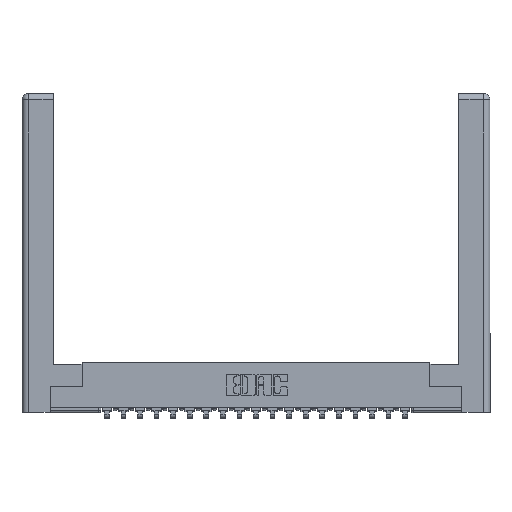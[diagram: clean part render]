
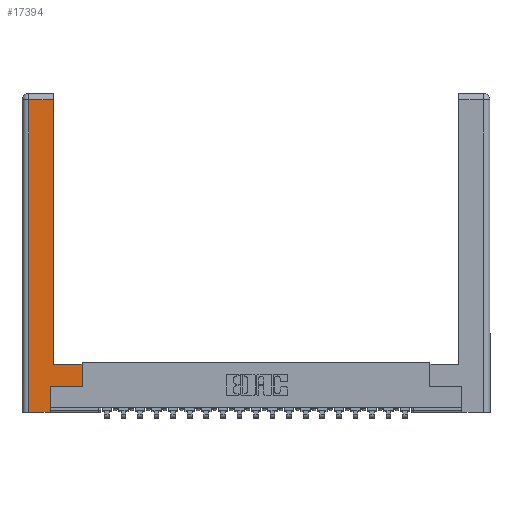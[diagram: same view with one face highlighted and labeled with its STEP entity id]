
A CAD part, top view. The second image highlights one B-rep face of the part: STEP entity #17394.
In plain terms, the highlighted planar face has unit normal (0, 0, 1).
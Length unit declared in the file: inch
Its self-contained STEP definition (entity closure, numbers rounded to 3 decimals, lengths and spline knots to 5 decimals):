
#299 = LINE ( 'NONE', #22290, #17505 ) ;
#764 = CARTESIAN_POINT ( 'NONE',  ( 0.565, 0.245, 0. ) ) ;
#1350 = EDGE_LOOP ( 'NONE', ( #5192, #10925, #2690, #4575, #13334, #8407, #13042, #10492 ) ) ;
#2161 = VERTEX_POINT ( 'NONE', #20354 ) ;
#2690 = ORIENTED_EDGE ( 'NONE', *, *, #7269, .T. ) ;
#3246 = LINE ( 'NONE', #17919, #8454 ) ;
#3253 = LINE ( 'NONE', #12446, #7632 ) ;
#3989 = EDGE_CURVE ( 'NONE', #17855, #9321, #9372, .T. ) ;
#4108 = DIRECTION ( 'NONE',  ( 0., 1., 0. ) ) ;
#4365 = CARTESIAN_POINT ( 'NONE',  ( 0.265, 0., 0. ) ) ;
#4575 = ORIENTED_EDGE ( 'NONE', *, *, #8338, .T. ) ;
#5192 = ORIENTED_EDGE ( 'NONE', *, *, #13053, .T. ) ;
#5226 = CARTESIAN_POINT ( 'NONE',  ( 0.265, 0., 0. ) ) ;
#6104 = CARTESIAN_POINT ( 'NONE',  ( 0.295, 0.45, 0. ) ) ;
#6985 = DIRECTION ( 'NONE',  ( 1., 0., 0. ) ) ;
#7269 = EDGE_CURVE ( 'NONE', #18601, #11705, #299, .T. ) ;
#7632 = VECTOR ( 'NONE', #8948, 39.37008 ) ;
#7721 = LINE ( 'NONE', #764, #10472 ) ;
#7973 = DIRECTION ( 'NONE',  ( 1., 0., 0. ) ) ;
#8338 = EDGE_CURVE ( 'NONE', #11705, #17855, #18162, .T. ) ;
#8407 = ORIENTED_EDGE ( 'NONE', *, *, #10264, .T. ) ;
#8454 = VECTOR ( 'NONE', #9273, 39.37008 ) ;
#8589 = VERTEX_POINT ( 'NONE', #6104 ) ;
#8853 = AXIS2_PLACEMENT_3D ( 'NONE', #20135, #11696, #18529 ) ;
#8880 = CARTESIAN_POINT ( 'NONE',  ( 0.0615, 2.94, 0. ) ) ;
#8948 = DIRECTION ( 'NONE',  ( 0., 1., 0. ) ) ;
#9206 = DIRECTION ( 'NONE',  ( 0., -1., 0. ) ) ;
#9273 = DIRECTION ( 'NONE',  ( 0., 1., 0. ) ) ;
#9319 = VECTOR ( 'NONE', #10439, 39.37008 ) ;
#9321 = VERTEX_POINT ( 'NONE', #18197 ) ;
#9372 = LINE ( 'NONE', #16461, #15376 ) ;
#10264 = EDGE_CURVE ( 'NONE', #9321, #13300, #7721, .T. ) ;
#10439 = DIRECTION ( 'NONE',  ( -1., 0., 0. ) ) ;
#10472 = VECTOR ( 'NONE', #7973, 39.37008 ) ;
#10492 = ORIENTED_EDGE ( 'NONE', *, *, #11711, .T. ) ;
#10714 = EDGE_CURVE ( 'NONE', #2161, #18601, #13141, .T. ) ;
#10776 = DIRECTION ( 'NONE',  ( -1., 0., 0. ) ) ;
#10829 = VECTOR ( 'NONE', #6985, 39.37008 ) ;
#10925 = ORIENTED_EDGE ( 'NONE', *, *, #10714, .T. ) ;
#11222 = VECTOR ( 'NONE', #10776, 39.37008 ) ;
#11696 = DIRECTION ( 'NONE',  ( 0., 0., -1. ) ) ;
#11705 = VERTEX_POINT ( 'NONE', #17585 ) ;
#11711 = EDGE_CURVE ( 'NONE', #14452, #8589, #19650, .T. ) ;
#12378 = CARTESIAN_POINT ( 'NONE',  ( 0.565, 0.45, 0. ) ) ;
#12446 = CARTESIAN_POINT ( 'NONE',  ( 0.565, 0.45, 0. ) ) ;
#13042 = ORIENTED_EDGE ( 'NONE', *, *, #20664, .T. ) ;
#13053 = EDGE_CURVE ( 'NONE', #8589, #2161, #3246, .T. ) ;
#13141 = LINE ( 'NONE', #8880, #11222 ) ;
#13300 = VERTEX_POINT ( 'NONE', #16161 ) ;
#13334 = ORIENTED_EDGE ( 'NONE', *, *, #3989, .T. ) ;
#13876 = CARTESIAN_POINT ( 'NONE',  ( 0.295, 0.45, 0. ) ) ;
#14452 = VERTEX_POINT ( 'NONE', #12378 ) ;
#15376 = VECTOR ( 'NONE', #4108, 39.37008 ) ;
#16161 = CARTESIAN_POINT ( 'NONE',  ( 0.565, 0.245, 0. ) ) ;
#16461 = CARTESIAN_POINT ( 'NONE',  ( 0.265, 0.245, 0. ) ) ;
#16724 = PLANE ( 'NONE',  #8853 ) ;
#17394 = ADVANCED_FACE ( 'NONE', ( #19166 ), #16724, .F. ) ;
#17505 = VECTOR ( 'NONE', #9206, 39.37008 ) ;
#17585 = CARTESIAN_POINT ( 'NONE',  ( 0.0615, 0., 0. ) ) ;
#17855 = VERTEX_POINT ( 'NONE', #4365 ) ;
#17919 = CARTESIAN_POINT ( 'NONE',  ( 0.295, 3., 0. ) ) ;
#18162 = LINE ( 'NONE', #5226, #10829 ) ;
#18197 = CARTESIAN_POINT ( 'NONE',  ( 0.265, 0.245, 0. ) ) ;
#18410 = CARTESIAN_POINT ( 'NONE',  ( 0.0615, 2.94, 0. ) ) ;
#18529 = DIRECTION ( 'NONE',  ( -1., 0., 0. ) ) ;
#18601 = VERTEX_POINT ( 'NONE', #18410 ) ;
#19166 = FACE_OUTER_BOUND ( 'NONE', #1350, .T. ) ;
#19650 = LINE ( 'NONE', #13876, #9319 ) ;
#20135 = CARTESIAN_POINT ( 'NONE',  ( 0., 0., 0. ) ) ;
#20354 = CARTESIAN_POINT ( 'NONE',  ( 0.295, 2.94, 0. ) ) ;
#20664 = EDGE_CURVE ( 'NONE', #13300, #14452, #3253, .T. ) ;
#22290 = CARTESIAN_POINT ( 'NONE',  ( 0.0615, 0., 0. ) ) ;
